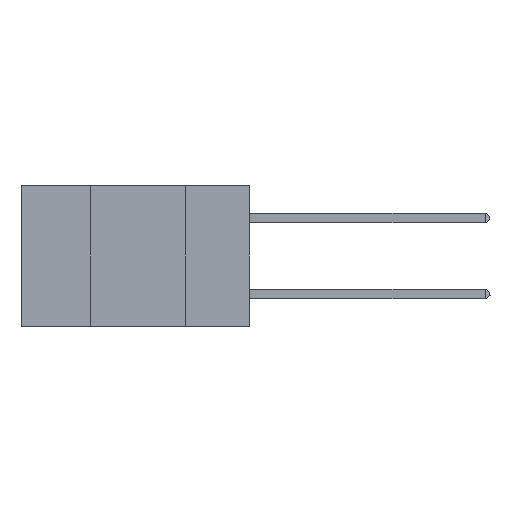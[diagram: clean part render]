
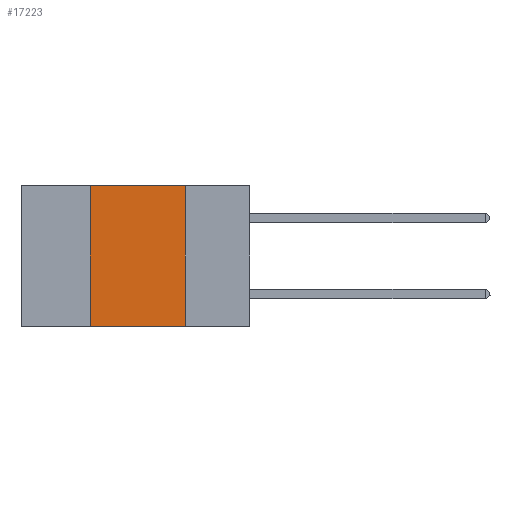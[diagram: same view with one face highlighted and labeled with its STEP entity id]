
A CAD part, left-side view. The second image highlights one B-rep face of the part: STEP entity #17223.
In plain terms, the highlighted planar face has unit normal (-1, 0, 0).
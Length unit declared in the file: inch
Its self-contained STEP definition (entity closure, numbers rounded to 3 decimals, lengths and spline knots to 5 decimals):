
#170 = CARTESIAN_POINT ( 'NONE',  ( 0., 0.17, -0.37 ) ) ;
#348 = EDGE_CURVE ( 'NONE', #8770, #17571, #13783, .T. ) ;
#1226 = CARTESIAN_POINT ( 'NONE',  ( 0., 0.6, -0.37 ) ) ;
#1806 = EDGE_CURVE ( 'NONE', #11749, #8770, #7277, .T. ) ;
#3107 = DIRECTION ( 'NONE',  ( 1., 0., 0. ) ) ;
#3446 = DIRECTION ( 'NONE',  ( 0., -1., 0. ) ) ;
#3624 = FACE_OUTER_BOUND ( 'NONE', #19849, .T. ) ;
#4672 = DIRECTION ( 'NONE',  ( 0., 0., -1. ) ) ;
#5040 = ORIENTED_EDGE ( 'NONE', *, *, #15189, .F. ) ;
#5451 = DIRECTION ( 'NONE',  ( 0., 0., 1. ) ) ;
#6519 = DIRECTION ( 'NONE',  ( 0., -1., 0. ) ) ;
#7064 = CARTESIAN_POINT ( 'NONE',  ( 0., 0.42, 0. ) ) ;
#7277 = LINE ( 'NONE', #16537, #20435 ) ;
#7598 = CARTESIAN_POINT ( 'NONE',  ( 0., 0.42, 0. ) ) ;
#7926 = CARTESIAN_POINT ( 'NONE',  ( 0., 0.6, 0. ) ) ;
#8686 = ORIENTED_EDGE ( 'NONE', *, *, #348, .F. ) ;
#8770 = VERTEX_POINT ( 'NONE', #19486 ) ;
#9358 = VECTOR ( 'NONE', #13895, 39.37008 ) ;
#10497 = EDGE_CURVE ( 'NONE', #19398, #17571, #16798, .T. ) ;
#11749 = VERTEX_POINT ( 'NONE', #7598 ) ;
#13455 = CARTESIAN_POINT ( 'NONE',  ( 0., 0.42, -0.37 ) ) ;
#13606 = CARTESIAN_POINT ( 'NONE',  ( 0., 0.17, 0. ) ) ;
#13783 = LINE ( 'NONE', #13606, #9358 ) ;
#13895 = DIRECTION ( 'NONE',  ( 0., 0., -1. ) ) ;
#15189 = EDGE_CURVE ( 'NONE', #19398, #11749, #16889, .T. ) ;
#15311 = VECTOR ( 'NONE', #5451, 39.37008 ) ;
#16208 = ORIENTED_EDGE ( 'NONE', *, *, #10497, .T. ) ;
#16537 = CARTESIAN_POINT ( 'NONE',  ( 0., 0.6, 0. ) ) ;
#16798 = LINE ( 'NONE', #1226, #20664 ) ;
#16889 = LINE ( 'NONE', #7064, #15311 ) ;
#17223 = ADVANCED_FACE ( 'NONE', ( #3624 ), #17903, .F. ) ;
#17571 = VERTEX_POINT ( 'NONE', #170 ) ;
#17903 = PLANE ( 'NONE',  #20304 ) ;
#19398 = VERTEX_POINT ( 'NONE', #13455 ) ;
#19486 = CARTESIAN_POINT ( 'NONE',  ( 0., 0.17, 0. ) ) ;
#19849 = EDGE_LOOP ( 'NONE', ( #8686, #21109, #5040, #16208 ) ) ;
#20304 = AXIS2_PLACEMENT_3D ( 'NONE', #7926, #3107, #4672 ) ;
#20435 = VECTOR ( 'NONE', #6519, 39.37008 ) ;
#20664 = VECTOR ( 'NONE', #3446, 39.37008 ) ;
#21109 = ORIENTED_EDGE ( 'NONE', *, *, #1806, .F. ) ;
